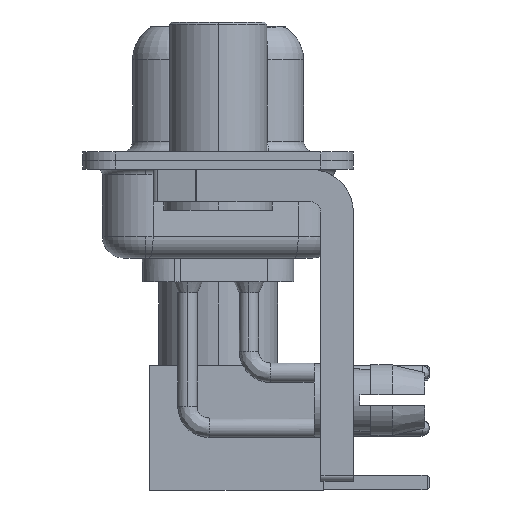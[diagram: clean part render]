
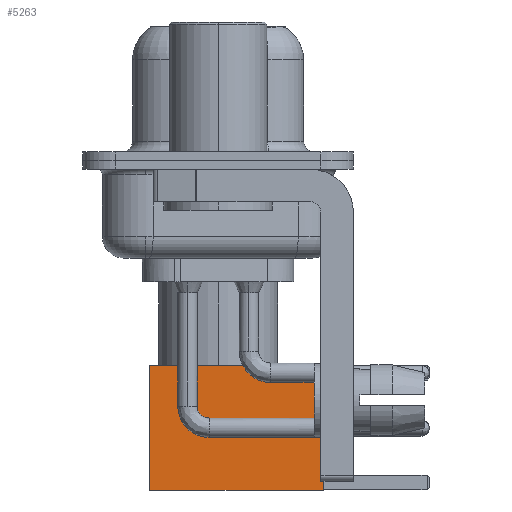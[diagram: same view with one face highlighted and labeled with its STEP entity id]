
A CAD part, left-side view. The second image highlights one B-rep face of the part: STEP entity #5263.
In plain terms, the highlighted face is planar.
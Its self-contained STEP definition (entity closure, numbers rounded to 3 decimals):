
#232 = VERTEX_POINT ( 'NONE', #17183 ) ;
#247 = LINE ( 'NONE', #21305, #2741 ) ;
#631 = VERTEX_POINT ( 'NONE', #20451 ) ;
#793 = CARTESIAN_POINT ( 'NONE',  ( -2.875, 2.875, 0. ) ) ;
#2645 = AXIS2_PLACEMENT_3D ( 'NONE', #11520, #9885, #18628 ) ;
#2741 = VECTOR ( 'NONE', #18025, 1000. ) ;
#2753 = CARTESIAN_POINT ( 'NONE',  ( -2.875, 2.875, 8. ) ) ;
#2814 = PLANE ( 'NONE',  #2645 ) ;
#3068 = VECTOR ( 'NONE', #13018, 1000. ) ;
#3487 = LINE ( 'NONE', #12521, #5691 ) ;
#5263 = ADVANCED_FACE ( 'NONE', ( #13240 ), #2814, .T. ) ;
#5691 = VECTOR ( 'NONE', #17996, 1000. ) ;
#6075 = CARTESIAN_POINT ( 'NONE',  ( 0., 2.875, 0. ) ) ;
#8581 = DIRECTION ( 'NONE',  ( 0., 0., -1. ) ) ;
#9885 = DIRECTION ( 'NONE',  ( 0., 1., 0. ) ) ;
#10322 = LINE ( 'NONE', #17415, #13432 ) ;
#11520 = CARTESIAN_POINT ( 'NONE',  ( 2.875, 2.875, 0. ) ) ;
#12521 = CARTESIAN_POINT ( 'NONE',  ( 2.875, 2.875, 0. ) ) ;
#13018 = DIRECTION ( 'NONE',  ( -1., 0., 0. ) ) ;
#13240 = FACE_OUTER_BOUND ( 'NONE', #16153, .T. ) ;
#13432 = VECTOR ( 'NONE', #8581, 1000. ) ;
#16153 = EDGE_LOOP ( 'NONE', ( #20457, #21211, #19407, #17210 ) ) ;
#16513 = LINE ( 'NONE', #6075, #3068 ) ;
#17183 = CARTESIAN_POINT ( 'NONE',  ( 2.875, 2.875, 8. ) ) ;
#17210 = ORIENTED_EDGE ( 'NONE', *, *, #21959, .F. ) ;
#17415 = CARTESIAN_POINT ( 'NONE',  ( -2.875, 2.875, 0. ) ) ;
#17996 = DIRECTION ( 'NONE',  ( 0., 0., -1. ) ) ;
#18025 = DIRECTION ( 'NONE',  ( -1., 0., 0. ) ) ;
#18037 = VERTEX_POINT ( 'NONE', #793 ) ;
#18628 = DIRECTION ( 'NONE',  ( 0., 0., 1. ) ) ;
#18919 = EDGE_CURVE ( 'NONE', #631, #18037, #16513, .T. ) ;
#19407 = ORIENTED_EDGE ( 'NONE', *, *, #20957, .F. ) ;
#19865 = VERTEX_POINT ( 'NONE', #2753 ) ;
#20451 = CARTESIAN_POINT ( 'NONE',  ( 2.875, 2.875, 0. ) ) ;
#20457 = ORIENTED_EDGE ( 'NONE', *, *, #21105, .T. ) ;
#20957 = EDGE_CURVE ( 'NONE', #19865, #18037, #10322, .T. ) ;
#21105 = EDGE_CURVE ( 'NONE', #232, #631, #3487, .T. ) ;
#21211 = ORIENTED_EDGE ( 'NONE', *, *, #18919, .T. ) ;
#21305 = CARTESIAN_POINT ( 'NONE',  ( 0., 2.875, 8. ) ) ;
#21959 = EDGE_CURVE ( 'NONE', #232, #19865, #247, .T. ) ;
